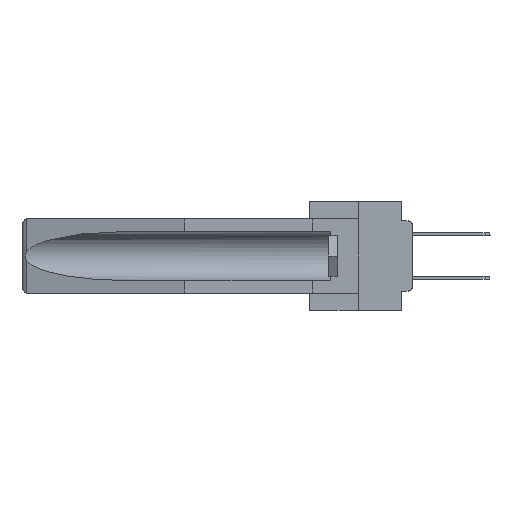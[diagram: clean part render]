
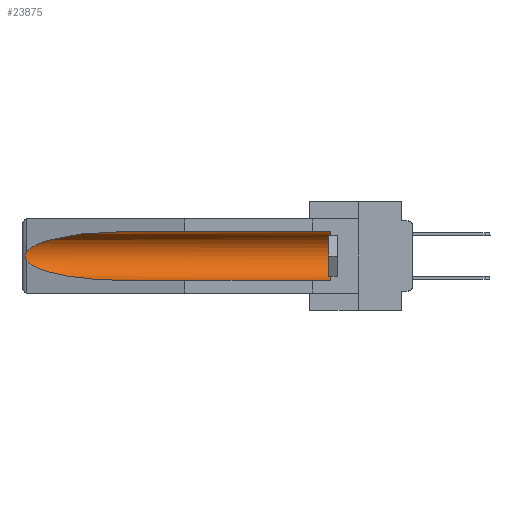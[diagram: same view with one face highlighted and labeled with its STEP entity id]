
A CAD part, left-side view. The second image highlights one B-rep face of the part: STEP entity #23875.
In plain terms, the highlighted cylindrical face has radius 2.857 mm (diameter 5.715 mm), a partial arc.
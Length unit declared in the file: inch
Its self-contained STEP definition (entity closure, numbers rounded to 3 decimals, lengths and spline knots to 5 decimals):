
#574 = CARTESIAN_POINT ( 'NONE',  ( 0.155, 0.126, -0.284 ) ) ;
#701 = EDGE_CURVE ( 'NONE', #12436, #24081, #28395, .T. ) ;
#866 = CARTESIAN_POINT ( 'NONE',  ( 0.26597, 1.5296, -0.19026 ) ) ;
#1728 = DIRECTION ( 'NONE',  ( 0., 1., 0. ) ) ;
#1803 = AXIS2_PLACEMENT_3D ( 'NONE', #17791, #13047, #34333 ) ;
#2320 = VERTEX_POINT ( 'NONE', #34811 ) ;
#2380 = CARTESIAN_POINT ( 'NONE',  ( 0.155, 0.126, -0.1715 ) ) ;
#2482 = ORIENTED_EDGE ( 'NONE', *, *, #19843, .T. ) ;
#3238 = CARTESIAN_POINT ( 'NONE',  ( 0.2673, 1.5327, -0.16383 ) ) ;
#4375 = CARTESIAN_POINT ( 'NONE',  ( 0.155, 0.126, -0.059 ) ) ;
#4642 = ORIENTED_EDGE ( 'NONE', *, *, #35882, .T. ) ;
#5956 = CIRCLE ( 'NONE', #13513, 0.1125 ) ;
#6344 = CARTESIAN_POINT ( 'NONE',  ( 0.26537, 1.52718, -0.14972 ) ) ;
#6717 = DIRECTION ( 'NONE',  ( 0., 1., 0. ) ) ;
#6775 = VERTEX_POINT ( 'NONE', #23937 ) ;
#7012 = LINE ( 'NONE', #29583, #24685 ) ;
#7100 = VECTOR ( 'NONE', #6717, 39.37008 ) ;
#7326 = CARTESIAN_POINT ( 'NONE',  ( 0.26537, 1.52718, -0.19328 ) ) ;
#7870 = CARTESIAN_POINT ( 'NONE',  ( 0.25451, 1.48313, -0.24835 ) ) ;
#8874 = CARTESIAN_POINT ( 'NONE',  ( 0.26654, 1.53092, -0.15636 ) ) ;
#8886 = EDGE_CURVE ( 'NONE', #32100, #2320, #33908, .T. ) ;
#9872 = CARTESIAN_POINT ( 'NONE',  ( 0.21114, 1.30732, -0.284 ) ) ;
#9994 = CARTESIAN_POINT ( 'NONE',  ( 0.21114, 1.30732, -0.059 ) ) ;
#11425 = VERTEX_POINT ( 'NONE', #4375 ) ;
#11977 = CARTESIAN_POINT ( 'NONE',  ( 0.26537, 1.52718, -0.19328 ) ) ;
#12365 = CARTESIAN_POINT ( 'NONE',  ( 0.26537, 1.52718, -0.14972 ) ) ;
#12436 = VERTEX_POINT ( 'NONE', #574 ) ;
#13047 = DIRECTION ( 'NONE',  ( 0., 1., 0. ) ) ;
#13484 = DIRECTION ( 'NONE',  ( 0., -1., 0. ) ) ;
#13513 = AXIS2_PLACEMENT_3D ( 'NONE', #2380, #13484, #24612 ) ;
#13691 = ORIENTED_EDGE ( 'NONE', *, *, #27528, .T. ) ;
#14707 = CARTESIAN_POINT ( 'NONE',  ( 0.2675, 1.53308, -0.17534 ) ) ;
#15242 = CYLINDRICAL_SURFACE ( 'NONE', #1803, 0.1125 ) ;
#15975 = CARTESIAN_POINT ( 'NONE',  ( 0.155, 1.07973, -0.284 ) ) ;
#16761 = B_SPLINE_CURVE_WITH_KNOTS ( 'NONE', 3,
 ( #6344, #30896, #8874, #3238, #20016, #14707, #31070, #25826, #866, #11977 ),
 .UNSPECIFIED., .F., .F.,
 ( 4, 2, 2, 2, 4 ),
 ( 0., 0.00029, 0.00058, 0.00087, 0.00117 ),
 .UNSPECIFIED. ) ;
#17698 = ORIENTED_EDGE ( 'NONE', *, *, #34227, .T. ) ;
#17791 = CARTESIAN_POINT ( 'NONE',  ( 0.155, -0.30754, -0.1715 ) ) ;
#19843 = EDGE_CURVE ( 'NONE', #2320, #6775, #16761, .T. ) ;
#20016 = CARTESIAN_POINT ( 'NONE',  ( 0.2675, 1.53308, -0.16763 ) ) ;
#23573 = ORIENTED_EDGE ( 'NONE', *, *, #8886, .T. ) ;
#23683 = EDGE_LOOP ( 'NONE', ( #23573, #2482, #4642, #29760, #13691, #17698 ) ) ;
#23875 = ADVANCED_FACE ( 'NONE', ( #26169 ), #15242, .F. ) ;
#23937 = CARTESIAN_POINT ( 'NONE',  ( 0.26537, 1.52718, -0.19328 ) ) ;
#24081 = VERTEX_POINT ( 'NONE', #15975 ) ;
#24612 = DIRECTION ( 'NONE',  ( 0., 0., 1. ) ) ;
#24685 = VECTOR ( 'NONE', #1728, 39.37008 ) ;
#25554 =( BOUNDED_CURVE ( )  B_SPLINE_CURVE ( 3, ( #7326, #7870, #9872, #26989 ),
 .UNSPECIFIED., .F., .F. ) 
 B_SPLINE_CURVE_WITH_KNOTS ( ( 4, 4 ),
 ( 0.1948, 1.5708 ),
 .UNSPECIFIED. ) 
 CURVE ( )  GEOMETRIC_REPRESENTATION_ITEM ( )  RATIONAL_B_SPLINE_CURVE ( ( 1., 0.848, 0.848, 1. ) ) 
 REPRESENTATION_ITEM ( '' )  );
#25826 = CARTESIAN_POINT ( 'NONE',  ( 0.26655, 1.53094, -0.18657 ) ) ;
#26169 = FACE_OUTER_BOUND ( 'NONE', #23683, .T. ) ;
#26206 = CARTESIAN_POINT ( 'NONE',  ( 0.155, 1.07973, -0.059 ) ) ;
#26989 = CARTESIAN_POINT ( 'NONE',  ( 0.155, 1.07973, -0.284 ) ) ;
#27528 = EDGE_CURVE ( 'NONE', #12436, #11425, #5956, .T. ) ;
#28395 = LINE ( 'NONE', #31463, #7100 ) ;
#29471 = CARTESIAN_POINT ( 'NONE',  ( 0.25451, 1.48313, -0.09465 ) ) ;
#29583 = CARTESIAN_POINT ( 'NONE',  ( 0.155, -0.30754, -0.059 ) ) ;
#29760 = ORIENTED_EDGE ( 'NONE', *, *, #701, .F. ) ;
#30896 = CARTESIAN_POINT ( 'NONE',  ( 0.26597, 1.52961, -0.15275 ) ) ;
#31070 = CARTESIAN_POINT ( 'NONE',  ( 0.2673, 1.53269, -0.17917 ) ) ;
#31463 = CARTESIAN_POINT ( 'NONE',  ( 0.155, -0.30754, -0.284 ) ) ;
#32100 = VERTEX_POINT ( 'NONE', #35099 ) ;
#33908 =( BOUNDED_CURVE ( )  B_SPLINE_CURVE ( 3, ( #26206, #9994, #29471, #12365 ),
 .UNSPECIFIED., .F., .T. ) 
 B_SPLINE_CURVE_WITH_KNOTS ( ( 4, 4 ),
 ( 4.71239, 6.08839 ),
 .UNSPECIFIED. ) 
 CURVE ( )  GEOMETRIC_REPRESENTATION_ITEM ( )  RATIONAL_B_SPLINE_CURVE ( ( 1., 0.848, 0.848, 1. ) ) 
 REPRESENTATION_ITEM ( '' )  );
#34227 = EDGE_CURVE ( 'NONE', #11425, #32100, #7012, .T. ) ;
#34333 = DIRECTION ( 'NONE',  ( 0., 0., 1. ) ) ;
#34811 = CARTESIAN_POINT ( 'NONE',  ( 0.26537, 1.52718, -0.14972 ) ) ;
#35099 = CARTESIAN_POINT ( 'NONE',  ( 0.155, 1.07973, -0.059 ) ) ;
#35882 = EDGE_CURVE ( 'NONE', #6775, #24081, #25554, .T. ) ;
